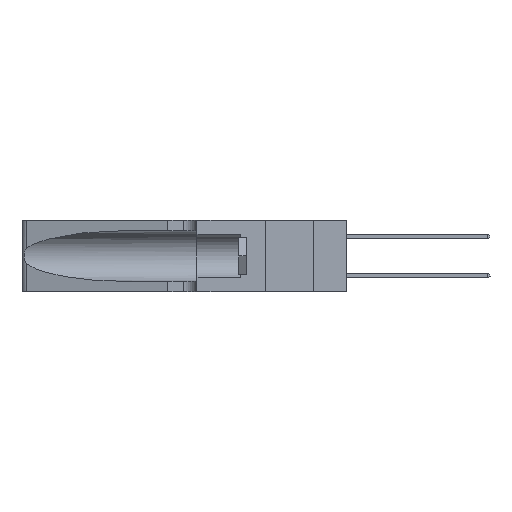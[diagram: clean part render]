
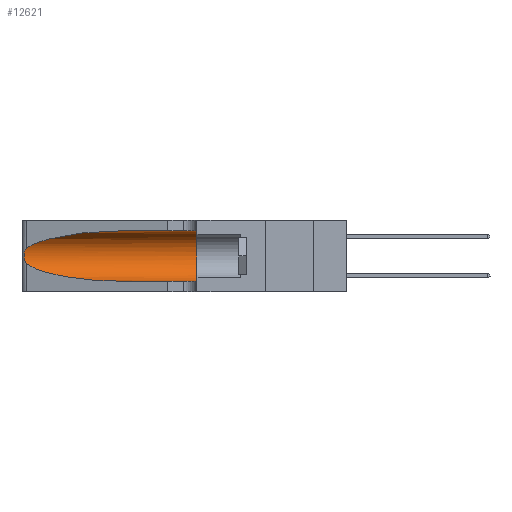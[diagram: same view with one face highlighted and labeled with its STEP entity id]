
A CAD part, left-side view. The second image highlights one B-rep face of the part: STEP entity #12621.
In plain terms, the highlighted cylindrical face has radius 3.308 mm (diameter 6.617 mm), a partial arc.
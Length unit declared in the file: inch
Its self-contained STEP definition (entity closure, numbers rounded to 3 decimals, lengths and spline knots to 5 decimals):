
#480 = CARTESIAN_POINT ( 'NONE',  ( 0.25487, 1.22718, 0.14631 ) ) ;
#3241 = CARTESIAN_POINT ( 'NONE',  ( 0.25487, 1.22718, 0.22369 ) ) ;
#3779 = ORIENTED_EDGE ( 'NONE', *, *, #7285, .T. ) ;
#4511 = CIRCLE ( 'NONE', #37854, 0.13025 ) ;
#6046 = CARTESIAN_POINT ( 'NONE',  ( 0.25856, 1.23593, 0.16098 ) ) ;
#6191 = DIRECTION ( 'NONE',  ( 0., 0., 1. ) ) ;
#6337 = CARTESIAN_POINT ( 'NONE',  ( 0.26018, 1.23835, 0.19895 ) ) ;
#6473 = CARTESIAN_POINT ( 'NONE',  ( 0.26075, 1.23896, 0.178 ) ) ;
#6543 =( BOUNDED_CURVE ( )  B_SPLINE_CURVE ( 3, ( #10142, #15450, #36563, #31097 ),
 .UNSPECIFIED., .F., .F. ) 
 B_SPLINE_CURVE_WITH_KNOTS ( ( 4, 4 ),
 ( 3.44316, 4.71239 ),
 .UNSPECIFIED. ) 
 CURVE ( )  GEOMETRIC_REPRESENTATION_ITEM ( )  RATIONAL_B_SPLINE_CURVE ( ( 1., 0.87, 0.87, 1. ) ) 
 REPRESENTATION_ITEM ( '' )  );
#6842 = CARTESIAN_POINT ( 'NONE',  ( 0.1305, 1.61858, 0.05475 ) ) ;
#7217 = DIRECTION ( 'NONE',  ( 0., -1., 0. ) ) ;
#7285 = EDGE_CURVE ( 'NONE', #33504, #40292, #6543, .T. ) ;
#8889 = VERTEX_POINT ( 'NONE', #32145 ) ;
#9478 = CARTESIAN_POINT ( 'NONE',  ( 0.1305, 0.35, 0.185 ) ) ;
#9594 = CARTESIAN_POINT ( 'NONE',  ( 0.2373, 1.15595, 0.28018 ) ) ;
#9619 = CARTESIAN_POINT ( 'NONE',  ( 0.25555, 1.22994, 0.2215 ) ) ;
#10142 = CARTESIAN_POINT ( 'NONE',  ( 0.25487, 1.22718, 0.14631 ) ) ;
#10372 = ORIENTED_EDGE ( 'NONE', *, *, #26630, .T. ) ;
#12621 = ADVANCED_FACE ( 'NONE', ( #31406 ), #26776, .F. ) ;
#12779 = DIRECTION ( 'NONE',  ( 0., 1., 0. ) ) ;
#13044 = CARTESIAN_POINT ( 'NONE',  ( 0.25487, 1.22718, 0.14631 ) ) ;
#13228 = CARTESIAN_POINT ( 'NONE',  ( 0.1305, 1.61858, 0.185 ) ) ;
#13302 = VECTOR ( 'NONE', #23377, 39.37008 ) ;
#13840 = CARTESIAN_POINT ( 'NONE',  ( 0.1305, 0.35, 0.05475 ) ) ;
#15450 = CARTESIAN_POINT ( 'NONE',  ( 0.2373, 1.15595, 0.08982 ) ) ;
#16173 = CARTESIAN_POINT ( 'NONE',  ( 0.25854, 1.2359, 0.20912 ) ) ;
#16480 = DIRECTION ( 'NONE',  ( 0., -1., 0. ) ) ;
#16696 = LINE ( 'NONE', #16917, #39789 ) ;
#16824 = LINE ( 'NONE', #6842, #13302 ) ;
#16917 = CARTESIAN_POINT ( 'NONE',  ( 0.1305, 1.61858, 0.31525 ) ) ;
#19041 = CARTESIAN_POINT ( 'NONE',  ( 0.25787, 1.23484, 0.2124 ) ) ;
#19295 = CARTESIAN_POINT ( 'NONE',  ( 0.18966, 0.96281, 0.31525 ) ) ;
#19317 = CARTESIAN_POINT ( 'NONE',  ( 0.25487, 1.22718, 0.22369 ) ) ;
#19465 = CARTESIAN_POINT ( 'NONE',  ( 0.25639, 1.23186, 0.15144 ) ) ;
#20613 = CARTESIAN_POINT ( 'NONE',  ( 0.25487, 1.22718, 0.22369 ) ) ;
#21621 = VERTEX_POINT ( 'NONE', #13840 ) ;
#21748 = B_SPLINE_CURVE_WITH_KNOTS ( 'NONE', 3,
 ( #19317, #9619, #35816, #19041, #16173, #6337, #32480, #6473, #22862, #6046, #39102, #19465, #42415, #13044 ),
 .UNSPECIFIED., .F., .F.,
 ( 4, 2, 2, 2, 2, 2, 4 ),
 ( 0., 0.00027, 0.00053, 0.00107, 0.0016, 0.00187, 0.00214 ),
 .UNSPECIFIED. ) ;
#22862 = CARTESIAN_POINT ( 'NONE',  ( 0.26017, 1.23833, 0.17102 ) ) ;
#23377 = DIRECTION ( 'NONE',  ( 0., -1., 0. ) ) ;
#23817 = ORIENTED_EDGE ( 'NONE', *, *, #31575, .F. ) ;
#24192 = EDGE_CURVE ( 'NONE', #26786, #35791, #42231, .T. ) ;
#26495 = DIRECTION ( 'NONE',  ( 0., 0., -1. ) ) ;
#26630 = EDGE_CURVE ( 'NONE', #40292, #21621, #16824, .T. ) ;
#26776 = CYLINDRICAL_SURFACE ( 'NONE', #31619, 0.13025 ) ;
#26786 = VERTEX_POINT ( 'NONE', #37765 ) ;
#31097 = CARTESIAN_POINT ( 'NONE',  ( 0.1305, 0.72297, 0.05475 ) ) ;
#31170 = EDGE_LOOP ( 'NONE', ( #39596, #36055, #3779, #10372, #23817, #32844 ) ) ;
#31406 = FACE_OUTER_BOUND ( 'NONE', #31170, .T. ) ;
#31575 = EDGE_CURVE ( 'NONE', #8889, #21621, #4511, .T. ) ;
#31619 = AXIS2_PLACEMENT_3D ( 'NONE', #13228, #16480, #26495 ) ;
#31673 = EDGE_CURVE ( 'NONE', #35791, #33504, #21748, .T. ) ;
#32145 = CARTESIAN_POINT ( 'NONE',  ( 0.1305, 0.35, 0.31525 ) ) ;
#32480 = CARTESIAN_POINT ( 'NONE',  ( 0.26075, 1.23896, 0.19203 ) ) ;
#32844 = ORIENTED_EDGE ( 'NONE', *, *, #37007, .F. ) ;
#32858 = CARTESIAN_POINT ( 'NONE',  ( 0.1305, 0.72297, 0.31525 ) ) ;
#33504 = VERTEX_POINT ( 'NONE', #480 ) ;
#35791 = VERTEX_POINT ( 'NONE', #20613 ) ;
#35816 = CARTESIAN_POINT ( 'NONE',  ( 0.25639, 1.23184, 0.21858 ) ) ;
#36055 = ORIENTED_EDGE ( 'NONE', *, *, #31673, .T. ) ;
#36563 = CARTESIAN_POINT ( 'NONE',  ( 0.18966, 0.96281, 0.05475 ) ) ;
#37007 = EDGE_CURVE ( 'NONE', #26786, #8889, #16696, .T. ) ;
#37765 = CARTESIAN_POINT ( 'NONE',  ( 0.1305, 0.72297, 0.31525 ) ) ;
#37854 = AXIS2_PLACEMENT_3D ( 'NONE', #9478, #12779, #6191 ) ;
#39102 = CARTESIAN_POINT ( 'NONE',  ( 0.25789, 1.23486, 0.15765 ) ) ;
#39596 = ORIENTED_EDGE ( 'NONE', *, *, #24192, .T. ) ;
#39789 = VECTOR ( 'NONE', #7217, 39.37008 ) ;
#40292 = VERTEX_POINT ( 'NONE', #40913 ) ;
#40913 = CARTESIAN_POINT ( 'NONE',  ( 0.1305, 0.72297, 0.05475 ) ) ;
#42231 =( BOUNDED_CURVE ( )  B_SPLINE_CURVE ( 3, ( #32858, #19295, #9594, #3241 ),
 .UNSPECIFIED., .F., .F. ) 
 B_SPLINE_CURVE_WITH_KNOTS ( ( 4, 4 ),
 ( 1.5708, 2.84003 ),
 .UNSPECIFIED. ) 
 CURVE ( )  GEOMETRIC_REPRESENTATION_ITEM ( )  RATIONAL_B_SPLINE_CURVE ( ( 1., 0.87, 0.87, 1. ) ) 
 REPRESENTATION_ITEM ( '' )  );
#42415 = CARTESIAN_POINT ( 'NONE',  ( 0.25555, 1.22993, 0.14849 ) ) ;
